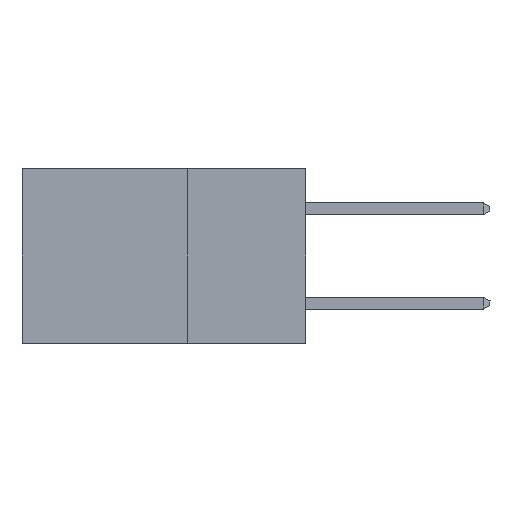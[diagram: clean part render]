
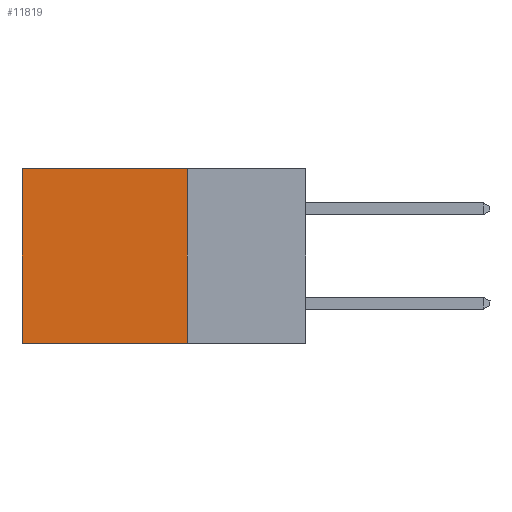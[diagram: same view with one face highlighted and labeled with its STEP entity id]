
A CAD part, left-side view. The second image highlights one B-rep face of the part: STEP entity #11819.
In plain terms, the highlighted planar face has unit normal (-1, 0, 0).
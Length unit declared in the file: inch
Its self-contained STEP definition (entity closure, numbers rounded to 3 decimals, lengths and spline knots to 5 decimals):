
#114 = CARTESIAN_POINT ( 'NONE',  ( 0.298, 0.6, -0.37 ) ) ;
#594 = ORIENTED_EDGE ( 'NONE', *, *, #635, .F. ) ;
#635 = EDGE_CURVE ( 'NONE', #960, #2947, #8573, .T. ) ;
#960 = VERTEX_POINT ( 'NONE', #3364 ) ;
#1389 = CARTESIAN_POINT ( 'NONE',  ( 0.298, 0.6, 0. ) ) ;
#1463 = LINE ( 'NONE', #11660, #1765 ) ;
#1765 = VECTOR ( 'NONE', #6446, 39.37008 ) ;
#2078 = ORIENTED_EDGE ( 'NONE', *, *, #11299, .T. ) ;
#2225 = VECTOR ( 'NONE', #9563, 39.37008 ) ;
#2947 = VERTEX_POINT ( 'NONE', #10651 ) ;
#2955 = CARTESIAN_POINT ( 'NONE',  ( 0.298, 0.25, 0. ) ) ;
#3364 = CARTESIAN_POINT ( 'NONE',  ( 0.298, 0.25, 0. ) ) ;
#3428 = FACE_OUTER_BOUND ( 'NONE', #3508, .T. ) ;
#3508 = EDGE_LOOP ( 'NONE', ( #2078, #7610, #594, #3959 ) ) ;
#3586 = DIRECTION ( 'NONE',  ( 0., 0., -1. ) ) ;
#3959 = ORIENTED_EDGE ( 'NONE', *, *, #8989, .T. ) ;
#3985 = EDGE_CURVE ( 'NONE', #2947, #4732, #1463, .T. ) ;
#4732 = VERTEX_POINT ( 'NONE', #114 ) ;
#6446 = DIRECTION ( 'NONE',  ( 0., 1., 0. ) ) ;
#7428 = LINE ( 'NONE', #11455, #9870 ) ;
#7610 = ORIENTED_EDGE ( 'NONE', *, *, #3985, .F. ) ;
#7673 = VECTOR ( 'NONE', #11070, 39.37008 ) ;
#7780 = CARTESIAN_POINT ( 'NONE',  ( 0.298, 0.6, 0. ) ) ;
#8573 = LINE ( 'NONE', #12286, #2225 ) ;
#8742 = PLANE ( 'NONE',  #9993 ) ;
#8989 = EDGE_CURVE ( 'NONE', #960, #9086, #7428, .T. ) ;
#9086 = VERTEX_POINT ( 'NONE', #7780 ) ;
#9510 = LINE ( 'NONE', #1389, #7673 ) ;
#9563 = DIRECTION ( 'NONE',  ( 0., 0., -1. ) ) ;
#9623 = DIRECTION ( 'NONE',  ( 0., 1., 0. ) ) ;
#9870 = VECTOR ( 'NONE', #9623, 39.37008 ) ;
#9993 = AXIS2_PLACEMENT_3D ( 'NONE', #2955, #10879, #3586 ) ;
#10651 = CARTESIAN_POINT ( 'NONE',  ( 0.298, 0.25, -0.37 ) ) ;
#10879 = DIRECTION ( 'NONE',  ( 1., 0., 0. ) ) ;
#11070 = DIRECTION ( 'NONE',  ( 0., 0., -1. ) ) ;
#11299 = EDGE_CURVE ( 'NONE', #9086, #4732, #9510, .T. ) ;
#11455 = CARTESIAN_POINT ( 'NONE',  ( 0.298, 0.25, 0. ) ) ;
#11660 = CARTESIAN_POINT ( 'NONE',  ( 0.298, 0.25, -0.37 ) ) ;
#11819 = ADVANCED_FACE ( 'NONE', ( #3428 ), #8742, .F. ) ;
#12286 = CARTESIAN_POINT ( 'NONE',  ( 0.298, 0.25, 0. ) ) ;
